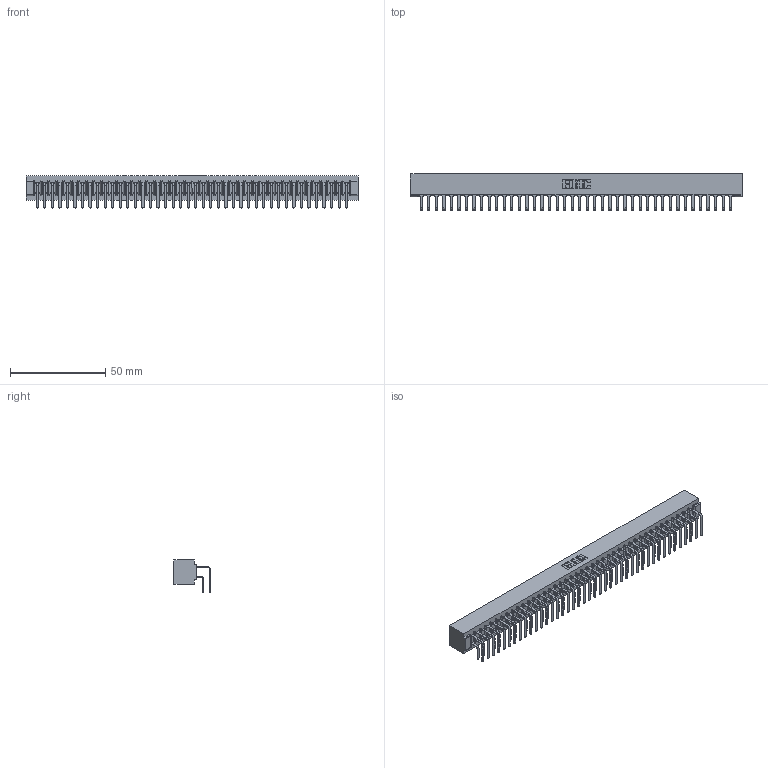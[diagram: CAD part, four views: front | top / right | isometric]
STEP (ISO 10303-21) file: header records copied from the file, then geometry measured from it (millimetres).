
FILE_DESCRIPTION (( 'STEP AP203' ), '1' );
FILE_NAME ('807-084-558-201.STEP', '2021-07-20T19:05:09', ( '' ), ( '' ), 'SwSTEP 2.0', 'SolidWorks 2020', '' );
FILE_SCHEMA (( 'CONFIG_CONTROL_DESIGN' ));
Length unit declared in the file: inch
Products named in the file (4): 807 Part_No Mounting Lugs; 307-290-001_558 - 2 (Single); 807-084-558-201; 307-290-001_558 559 - 1 (Single)
Assembly tree (85 placements, depth 2):
  807-084-558-201
    807 Part_No Mounting Lugs
    307-290-001_558 559 - 1 (Single)  x42
    307-290-001_558 - 2 (Single)  x42
Bounding box: 174.29 x 18.96 x 16.8 mm (x, y, z)
Volume: 19454.2 mm3; surface area: 26287.6 mm2
Topology: 85 solids, 85 shells, 4353 faces, 12227 edges, 7922 vertices
Faces by surface type: plane 2838, cylinder 1429, sphere 86
Entity records: 38519 total; most frequent: CARTESIAN_POINT 6300, ORIENTED_EDGE 6242, DIRECTION 6169, EDGE_CURVE 3121, VECTOR 2395, LINE 2395, VERTEX_POINT 2018, AXIS2_PLACEMENT_3D 1887
